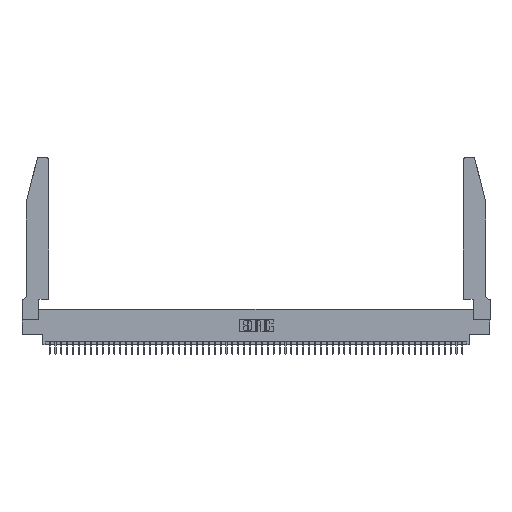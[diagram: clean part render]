
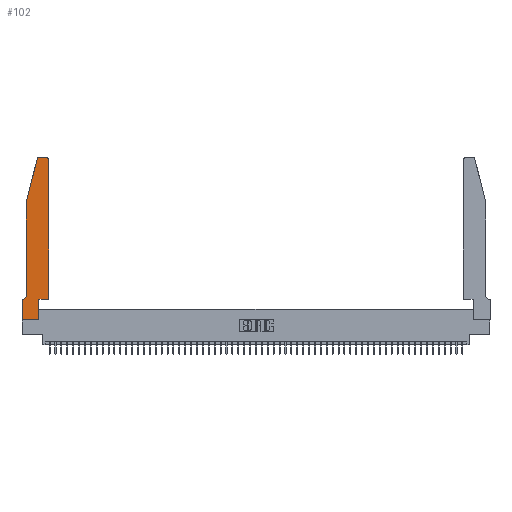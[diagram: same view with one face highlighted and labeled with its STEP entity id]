
A CAD part, top view. The second image highlights one B-rep face of the part: STEP entity #102.
In plain terms, the highlighted planar face has unit normal (0, 0, 1).
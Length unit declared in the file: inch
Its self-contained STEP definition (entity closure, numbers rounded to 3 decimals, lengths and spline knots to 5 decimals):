
#102 = ADVANCED_FACE ( 'NONE', ( #3974 ), #421, .T. ) ;
#228 = LINE ( 'NONE', #29092, #20804 ) ;
#421 = PLANE ( 'NONE',  #1890 ) ;
#532 = ORIENTED_EDGE ( 'NONE', *, *, #29567, .T. ) ;
#1059 = ORIENTED_EDGE ( 'NONE', *, *, #30776, .T. ) ;
#1760 = DIRECTION ( 'NONE',  ( 0., 1., 0. ) ) ;
#1770 = VECTOR ( 'NONE', #32088, 39.37008 ) ;
#1890 = AXIS2_PLACEMENT_3D ( 'NONE', #35518, #9266, #39906 ) ;
#1922 = LINE ( 'NONE', #24030, #23849 ) ;
#2056 = VERTEX_POINT ( 'NONE', #53977 ) ;
#2335 = ORIENTED_EDGE ( 'NONE', *, *, #49932, .T. ) ;
#2552 = DIRECTION ( 'NONE',  ( 0., 0., 1. ) ) ;
#2877 = DIRECTION ( 'NONE',  ( 0., 0., -1. ) ) ;
#3771 = CARTESIAN_POINT ( 'NONE',  ( 0.284, 2.75, 0.37 ) ) ;
#3974 = FACE_OUTER_BOUND ( 'NONE', #10109, .T. ) ;
#4391 = CARTESIAN_POINT ( 'NONE',  ( 0., 0., 0.37 ) ) ;
#6602 = LINE ( 'NONE', #54281, #27156 ) ;
#7514 = VERTEX_POINT ( 'NONE', #29019 ) ;
#7520 = LINE ( 'NONE', #4391, #10253 ) ;
#8866 = ORIENTED_EDGE ( 'NONE', *, *, #43014, .T. ) ;
#9068 = VERTEX_POINT ( 'NONE', #3771 ) ;
#9266 = DIRECTION ( 'NONE',  ( 0., 0., 1. ) ) ;
#9454 = VERTEX_POINT ( 'NONE', #16177 ) ;
#10048 = CARTESIAN_POINT ( 'NONE',  ( 0.0755, 2., 0.37 ) ) ;
#10109 = EDGE_LOOP ( 'NONE', ( #31150, #11919, #532, #42086, #11417, #1059, #44096, #40352, #42102, #2335, #8866, #49612 ) ) ;
#10195 = EDGE_CURVE ( 'NONE', #46930, #40880, #7520, .T. ) ;
#10253 = VECTOR ( 'NONE', #34884, 39.37008 ) ;
#11417 = ORIENTED_EDGE ( 'NONE', *, *, #32159, .T. ) ;
#11919 = ORIENTED_EDGE ( 'NONE', *, *, #12873, .T. ) ;
#12873 = EDGE_CURVE ( 'NONE', #9068, #2056, #34669, .T. ) ;
#13438 = VECTOR ( 'NONE', #14652, 39.37008 ) ;
#14001 = VECTOR ( 'NONE', #30601, 39.37008 ) ;
#14652 = DIRECTION ( 'NONE',  ( 0., -1., 0. ) ) ;
#15723 = CARTESIAN_POINT ( 'NONE',  ( 0.0755, 0.42, 0.37 ) ) ;
#16177 = CARTESIAN_POINT ( 'NONE',  ( 0.4505, 0.35, 0.37 ) ) ;
#16948 = AXIS2_PLACEMENT_3D ( 'NONE', #28812, #2552, #33258 ) ;
#20804 = VECTOR ( 'NONE', #46541, 39.37008 ) ;
#23262 = AXIS2_PLACEMENT_3D ( 'NONE', #29147, #2877, #33567 ) ;
#23581 = VECTOR ( 'NONE', #37706, 39.37008 ) ;
#23849 = VECTOR ( 'NONE', #28485, 39.37008 ) ;
#23858 = CARTESIAN_POINT ( 'NONE',  ( 0.284, 2.72, 0.37 ) ) ;
#24030 = CARTESIAN_POINT ( 'NONE',  ( 0.2605, 2.75, 0.37 ) ) ;
#24605 = CARTESIAN_POINT ( 'NONE',  ( 0., 0., 0.37 ) ) ;
#25093 = LINE ( 'NONE', #36479, #1770 ) ;
#26338 = EDGE_CURVE ( 'NONE', #47065, #46930, #25093, .T. ) ;
#27156 = VECTOR ( 'NONE', #1760, 39.37008 ) ;
#28299 = DIRECTION ( 'NONE',  ( 1., 0., 0. ) ) ;
#28485 = DIRECTION ( 'NONE',  ( -1., 0., 0. ) ) ;
#28812 = CARTESIAN_POINT ( 'NONE',  ( 0.4205, 2.72, 0.37 ) ) ;
#29019 = CARTESIAN_POINT ( 'NONE',  ( 0.0055, 0.35, 0.37 ) ) ;
#29092 = CARTESIAN_POINT ( 'NONE',  ( 0.0755, 0.35, 0.37 ) ) ;
#29147 = CARTESIAN_POINT ( 'NONE',  ( 0.0055, 0.42, 0.37 ) ) ;
#29225 = LINE ( 'NONE', #10048, #13438 ) ;
#29567 = EDGE_CURVE ( 'NONE', #2056, #43260, #49689, .T. ) ;
#29865 = VERTEX_POINT ( 'NONE', #43807 ) ;
#30601 = DIRECTION ( 'NONE',  ( 1., 0., 0. ) ) ;
#30776 = EDGE_CURVE ( 'NONE', #7514, #47065, #228, .T. ) ;
#30898 = LINE ( 'NONE', #43935, #41155 ) ;
#30903 = DIRECTION ( 'NONE',  ( 0., 1., 0. ) ) ;
#31150 = ORIENTED_EDGE ( 'NONE', *, *, #46852, .T. ) ;
#32088 = DIRECTION ( 'NONE',  ( 0., -1., 0. ) ) ;
#32159 = EDGE_CURVE ( 'NONE', #49011, #7514, #55632, .T. ) ;
#33258 = DIRECTION ( 'NONE',  ( 1., 0., 0. ) ) ;
#33567 = DIRECTION ( 'NONE',  ( -1., 0., 0. ) ) ;
#33686 = VERTEX_POINT ( 'NONE', #45905 ) ;
#34669 = CIRCLE ( 'NONE', #51079, 0.03 ) ;
#34884 = DIRECTION ( 'NONE',  ( 1., 0., 0. ) ) ;
#35518 = CARTESIAN_POINT ( 'NONE',  ( 0., 0.35, 0.37 ) ) ;
#36479 = CARTESIAN_POINT ( 'NONE',  ( 0., 0., 0.37 ) ) ;
#37706 = DIRECTION ( 'NONE',  ( -0.239, -0.971, 0. ) ) ;
#39232 = CARTESIAN_POINT ( 'NONE',  ( 0.4505, 0.35, 0.37 ) ) ;
#39906 = DIRECTION ( 'NONE',  ( 1., 0., 0. ) ) ;
#40352 = ORIENTED_EDGE ( 'NONE', *, *, #10195, .T. ) ;
#40390 = EDGE_CURVE ( 'NONE', #43260, #49011, #29225, .T. ) ;
#40811 = EDGE_CURVE ( 'NONE', #40880, #52095, #30898, .T. ) ;
#40880 = VERTEX_POINT ( 'NONE', #48713 ) ;
#41155 = VECTOR ( 'NONE', #30903, 39.37008 ) ;
#42086 = ORIENTED_EDGE ( 'NONE', *, *, #40390, .T. ) ;
#42102 = ORIENTED_EDGE ( 'NONE', *, *, #40811, .T. ) ;
#43014 = EDGE_CURVE ( 'NONE', #9454, #33686, #6602, .T. ) ;
#43260 = VERTEX_POINT ( 'NONE', #46818 ) ;
#43807 = CARTESIAN_POINT ( 'NONE',  ( 0.4205, 2.75, 0.37 ) ) ;
#43935 = CARTESIAN_POINT ( 'NONE',  ( 0.2865, 0.35, 0.37 ) ) ;
#44096 = ORIENTED_EDGE ( 'NONE', *, *, #26338, .T. ) ;
#44824 = CARTESIAN_POINT ( 'NONE',  ( 0.2865, 0.35, 0.37 ) ) ;
#45905 = CARTESIAN_POINT ( 'NONE',  ( 0.4505, 2.72, 0.37 ) ) ;
#46541 = DIRECTION ( 'NONE',  ( -1., 0., 0. ) ) ;
#46818 = CARTESIAN_POINT ( 'NONE',  ( 0.0755, 2., 0.37 ) ) ;
#46852 = EDGE_CURVE ( 'NONE', #29865, #9068, #1922, .T. ) ;
#46930 = VERTEX_POINT ( 'NONE', #24605 ) ;
#47065 = VERTEX_POINT ( 'NONE', #56249 ) ;
#48452 = EDGE_CURVE ( 'NONE', #33686, #29865, #56618, .T. ) ;
#48713 = CARTESIAN_POINT ( 'NONE',  ( 0.2865, 0., 0.37 ) ) ;
#48976 = LINE ( 'NONE', #39232, #14001 ) ;
#49011 = VERTEX_POINT ( 'NONE', #15723 ) ;
#49612 = ORIENTED_EDGE ( 'NONE', *, *, #48452, .T. ) ;
#49689 = LINE ( 'NONE', #50772, #23581 ) ;
#49932 = EDGE_CURVE ( 'NONE', #52095, #9454, #48976, .T. ) ;
#50772 = CARTESIAN_POINT ( 'NONE',  ( 0.0755, 2., 0.37 ) ) ;
#51079 = AXIS2_PLACEMENT_3D ( 'NONE', #23858, #54568, #28299 ) ;
#52095 = VERTEX_POINT ( 'NONE', #44824 ) ;
#53977 = CARTESIAN_POINT ( 'NONE',  ( 0.25487, 2.72718, 0.37 ) ) ;
#54281 = CARTESIAN_POINT ( 'NONE',  ( 0.4505, 0.35, 0.37 ) ) ;
#54568 = DIRECTION ( 'NONE',  ( 0., 0., 1. ) ) ;
#55632 = CIRCLE ( 'NONE', #23262, 0.07 ) ;
#56249 = CARTESIAN_POINT ( 'NONE',  ( 0., 0.35, 0.37 ) ) ;
#56618 = CIRCLE ( 'NONE', #16948, 0.03 ) ;
